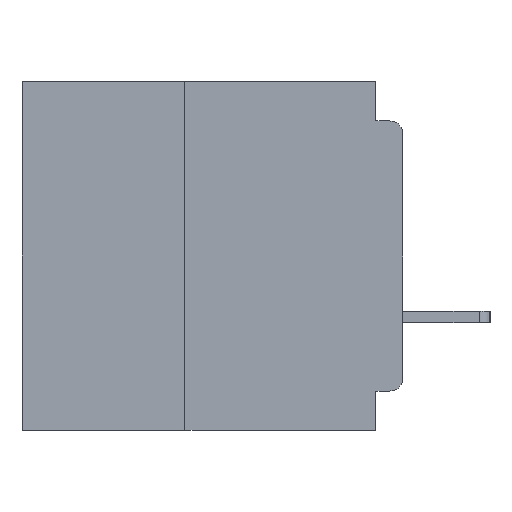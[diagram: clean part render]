
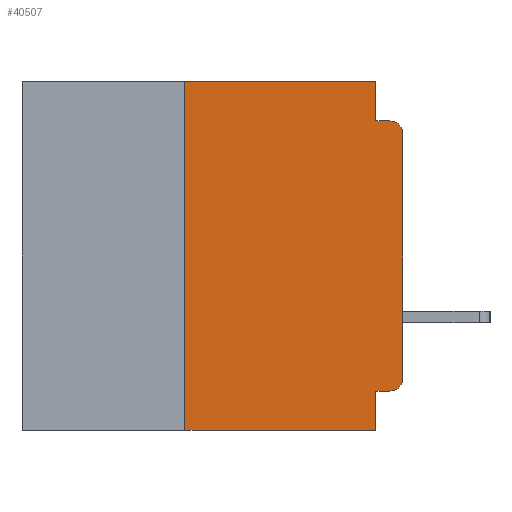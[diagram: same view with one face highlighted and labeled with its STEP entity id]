
A CAD part, left-side view. The second image highlights one B-rep face of the part: STEP entity #40507.
In plain terms, the highlighted planar face has unit normal (-1, 0, 0).
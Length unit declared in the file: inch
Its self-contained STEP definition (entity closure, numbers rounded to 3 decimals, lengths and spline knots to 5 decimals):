
#267 = VECTOR ( 'NONE', #41262, 39.37008 ) ;
#764 = VERTEX_POINT ( 'NONE', #19750 ) ;
#1232 = DIRECTION ( 'NONE',  ( 0., 0., -1. ) ) ;
#3643 = AXIS2_PLACEMENT_3D ( 'NONE', #40203, #18398, #43879 ) ;
#5584 = EDGE_CURVE ( 'NONE', #36960, #28611, #22084, .T. ) ;
#6875 = ORIENTED_EDGE ( 'NONE', *, *, #5584, .F. ) ;
#7413 = EDGE_CURVE ( 'NONE', #42217, #31674, #15718, .T. ) ;
#7493 = CARTESIAN_POINT ( 'NONE',  ( 0., 0.031, 0. ) ) ;
#8614 = ORIENTED_EDGE ( 'NONE', *, *, #46545, .F. ) ;
#10086 = LINE ( 'NONE', #12058, #267 ) ;
#11375 = VECTOR ( 'NONE', #28405, 39.37008 ) ;
#11882 = DIRECTION ( 'NONE',  ( -1., 0., 0. ) ) ;
#12058 = CARTESIAN_POINT ( 'NONE',  ( 0., 0., 0. ) ) ;
#14721 = PLANE ( 'NONE',  #3643 ) ;
#15162 = CARTESIAN_POINT ( 'NONE',  ( 0., 0.031, 0. ) ) ;
#15401 = LINE ( 'NONE', #23868, #33608 ) ;
#15516 = CIRCLE ( 'NONE', #28925, 0.015 ) ;
#15718 = LINE ( 'NONE', #34441, #26506 ) ;
#16313 = DIRECTION ( 'NONE',  ( 0., 1., 0. ) ) ;
#16668 = ORIENTED_EDGE ( 'NONE', *, *, #31615, .F. ) ;
#17420 = CARTESIAN_POINT ( 'NONE',  ( 0., 0.031, -0.4 ) ) ;
#18398 = DIRECTION ( 'NONE',  ( 1., 0., 0. ) ) ;
#18830 = DIRECTION ( 'NONE',  ( 0., 0., -1. ) ) ;
#19438 = EDGE_CURVE ( 'NONE', #31674, #46198, #30424, .T. ) ;
#19750 = CARTESIAN_POINT ( 'NONE',  ( 0., 0.25, -0.4 ) ) ;
#19819 = VECTOR ( 'NONE', #22758, 39.37008 ) ;
#20562 = CARTESIAN_POINT ( 'NONE',  ( 0., 0.031, -0.355 ) ) ;
#20618 = EDGE_CURVE ( 'NONE', #42217, #28420, #15516, .T. ) ;
#21076 = CARTESIAN_POINT ( 'NONE',  ( 0., 0., -0.045 ) ) ;
#21099 = CARTESIAN_POINT ( 'NONE',  ( 0., 0.015, -0.355 ) ) ;
#21222 = DIRECTION ( 'NONE',  ( 0., 0., -1. ) ) ;
#21403 = ORIENTED_EDGE ( 'NONE', *, *, #7413, .F. ) ;
#21476 = CARTESIAN_POINT ( 'NONE',  ( 0., 0.25, 0. ) ) ;
#21877 = AXIS2_PLACEMENT_3D ( 'NONE', #33719, #11882, #37412 ) ;
#22084 = LINE ( 'NONE', #30075, #19819 ) ;
#22358 = ORIENTED_EDGE ( 'NONE', *, *, #26722, .T. ) ;
#22516 = CARTESIAN_POINT ( 'NONE',  ( 0., 0.031, -0.4 ) ) ;
#22758 = DIRECTION ( 'NONE',  ( 0., -1., 0. ) ) ;
#23186 = DIRECTION ( 'NONE',  ( -1., 0., 0. ) ) ;
#23868 = CARTESIAN_POINT ( 'NONE',  ( 0., 0.25, -0.4 ) ) ;
#24514 = LINE ( 'NONE', #24747, #11375 ) ;
#24664 = VECTOR ( 'NONE', #42899, 39.37008 ) ;
#24747 = CARTESIAN_POINT ( 'NONE',  ( 0., 0.437, -0.4 ) ) ;
#25814 = LINE ( 'NONE', #21076, #24664 ) ;
#26506 = VECTOR ( 'NONE', #16313, 39.37008 ) ;
#26722 = EDGE_CURVE ( 'NONE', #764, #46198, #24514, .T. ) ;
#27407 = ORIENTED_EDGE ( 'NONE', *, *, #33424, .T. ) ;
#27444 = VERTEX_POINT ( 'NONE', #33307 ) ;
#27531 = DIRECTION ( 'NONE',  ( 0., 0., 1. ) ) ;
#28405 = DIRECTION ( 'NONE',  ( 0., -1., 0. ) ) ;
#28420 = VERTEX_POINT ( 'NONE', #39132 ) ;
#28611 = VERTEX_POINT ( 'NONE', #7493 ) ;
#28925 = AXIS2_PLACEMENT_3D ( 'NONE', #45027, #23186, #1232 ) ;
#29268 = VECTOR ( 'NONE', #21222, 39.37008 ) ;
#30075 = CARTESIAN_POINT ( 'NONE',  ( 0., 0.437, 0. ) ) ;
#30424 = LINE ( 'NONE', #17420, #29268 ) ;
#31615 = EDGE_CURVE ( 'NONE', #764, #36960, #15401, .T. ) ;
#31674 = VERTEX_POINT ( 'NONE', #20562 ) ;
#32748 = LINE ( 'NONE', #15162, #39046 ) ;
#33102 = VERTEX_POINT ( 'NONE', #35842 ) ;
#33307 = CARTESIAN_POINT ( 'NONE',  ( 0., 0., -0.06 ) ) ;
#33424 = EDGE_CURVE ( 'NONE', #28420, #27444, #10086, .T. ) ;
#33551 = CARTESIAN_POINT ( 'NONE',  ( 0., 0.031, -0.045 ) ) ;
#33608 = VECTOR ( 'NONE', #27531, 39.37008 ) ;
#33719 = CARTESIAN_POINT ( 'NONE',  ( 0., 0.015, -0.06 ) ) ;
#34441 = CARTESIAN_POINT ( 'NONE',  ( 0., 0., -0.355 ) ) ;
#34477 = FACE_OUTER_BOUND ( 'NONE', #40644, .T. ) ;
#35263 = EDGE_CURVE ( 'NONE', #27444, #33102, #42781, .T. ) ;
#35842 = CARTESIAN_POINT ( 'NONE',  ( 0., 0.015, -0.045 ) ) ;
#36960 = VERTEX_POINT ( 'NONE', #21476 ) ;
#37412 = DIRECTION ( 'NONE',  ( 0., 0., -1. ) ) ;
#38968 = EDGE_CURVE ( 'NONE', #28611, #39576, #32748, .T. ) ;
#39046 = VECTOR ( 'NONE', #18830, 39.37008 ) ;
#39132 = CARTESIAN_POINT ( 'NONE',  ( 0., 0., -0.34 ) ) ;
#39576 = VERTEX_POINT ( 'NONE', #33551 ) ;
#40203 = CARTESIAN_POINT ( 'NONE',  ( 0., 0.437, 0. ) ) ;
#40247 = ORIENTED_EDGE ( 'NONE', *, *, #20618, .T. ) ;
#40507 = ADVANCED_FACE ( 'NONE', ( #34477 ), #14721, .F. ) ;
#40644 = EDGE_LOOP ( 'NONE', ( #27407, #42866, #8614, #47368, #6875, #16668, #22358, #44166, #21403, #40247 ) ) ;
#41262 = DIRECTION ( 'NONE',  ( 0., 0., 1. ) ) ;
#42217 = VERTEX_POINT ( 'NONE', #21099 ) ;
#42781 = CIRCLE ( 'NONE', #21877, 0.015 ) ;
#42866 = ORIENTED_EDGE ( 'NONE', *, *, #35263, .T. ) ;
#42899 = DIRECTION ( 'NONE',  ( 0., -1., 0. ) ) ;
#43879 = DIRECTION ( 'NONE',  ( 0., 0., -1. ) ) ;
#44166 = ORIENTED_EDGE ( 'NONE', *, *, #19438, .F. ) ;
#45027 = CARTESIAN_POINT ( 'NONE',  ( 0., 0.015, -0.34 ) ) ;
#46198 = VERTEX_POINT ( 'NONE', #22516 ) ;
#46545 = EDGE_CURVE ( 'NONE', #39576, #33102, #25814, .T. ) ;
#47368 = ORIENTED_EDGE ( 'NONE', *, *, #38968, .F. ) ;
